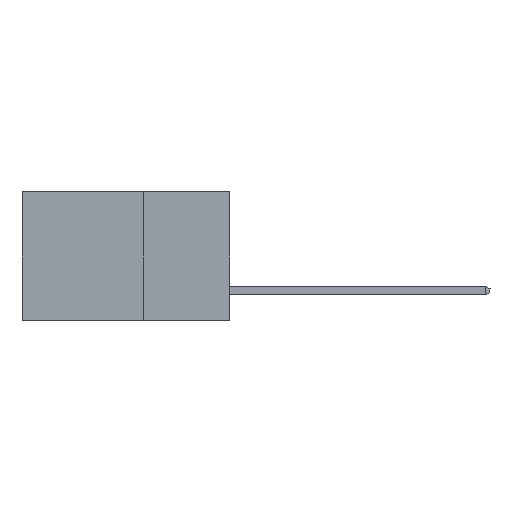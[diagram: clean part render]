
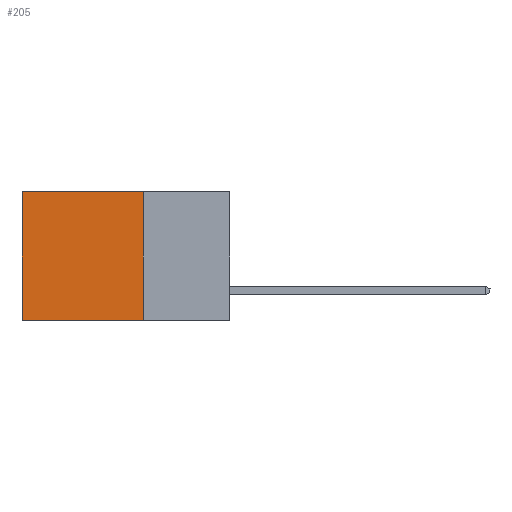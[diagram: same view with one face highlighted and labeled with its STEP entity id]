
A CAD part, left-side view. The second image highlights one B-rep face of the part: STEP entity #205.
In plain terms, the highlighted planar face has unit normal (-1, 0, 0).
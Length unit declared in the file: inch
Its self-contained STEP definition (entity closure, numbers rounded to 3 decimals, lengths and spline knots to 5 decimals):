
#205 = ADVANCED_FACE ( 'NONE', ( #17928 ), #16292, .F. ) ;
#658 = DIRECTION ( 'NONE',  ( 0., 0., -1. ) ) ;
#1501 = ORIENTED_EDGE ( 'NONE', *, *, #4145, .T. ) ;
#1997 = LINE ( 'NONE', #7866, #11590 ) ;
#3904 = LINE ( 'NONE', #15305, #12214 ) ;
#4145 = EDGE_CURVE ( 'NONE', #8951, #12545, #3904, .T. ) ;
#4415 = DIRECTION ( 'NONE',  ( 0., 1., 0. ) ) ;
#4969 = EDGE_CURVE ( 'NONE', #8951, #15960, #1997, .T. ) ;
#5435 = EDGE_CURVE ( 'NONE', #12545, #11303, #9252, .T. ) ;
#6039 = VECTOR ( 'NONE', #4415, 39.37008 ) ;
#6071 = CARTESIAN_POINT ( 'NONE',  ( 0.2615, 0.6, -0.37 ) ) ;
#6176 = CARTESIAN_POINT ( 'NONE',  ( 0.2615, 0.25, -0.37 ) ) ;
#6348 = DIRECTION ( 'NONE',  ( 0., 0., -1. ) ) ;
#7554 = CARTESIAN_POINT ( 'NONE',  ( 0.2615, 0.6, -0.37 ) ) ;
#7866 = CARTESIAN_POINT ( 'NONE',  ( 0.2615, 0.25, -0.37 ) ) ;
#8060 = VECTOR ( 'NONE', #15090, 39.37008 ) ;
#8951 = VERTEX_POINT ( 'NONE', #13808 ) ;
#9252 = LINE ( 'NONE', #7554, #8060 ) ;
#9755 = DIRECTION ( 'NONE',  ( 0., 1., 0. ) ) ;
#10037 = ORIENTED_EDGE ( 'NONE', *, *, #15325, .F. ) ;
#10166 = LINE ( 'NONE', #14853, #6039 ) ;
#11303 = VERTEX_POINT ( 'NONE', #6071 ) ;
#11590 = VECTOR ( 'NONE', #658, 39.37008 ) ;
#11899 = CARTESIAN_POINT ( 'NONE',  ( 0.2615, 0.6, 0. ) ) ;
#12176 = CARTESIAN_POINT ( 'NONE',  ( 0.2615, 0.25, -0.37 ) ) ;
#12214 = VECTOR ( 'NONE', #9755, 39.37008 ) ;
#12545 = VERTEX_POINT ( 'NONE', #11899 ) ;
#13386 = EDGE_LOOP ( 'NONE', ( #18352, #10037, #14983, #1501 ) ) ;
#13808 = CARTESIAN_POINT ( 'NONE',  ( 0.2615, 0.25, 0. ) ) ;
#14853 = CARTESIAN_POINT ( 'NONE',  ( 0.2615, 0.25, -0.37 ) ) ;
#14983 = ORIENTED_EDGE ( 'NONE', *, *, #4969, .F. ) ;
#15090 = DIRECTION ( 'NONE',  ( 0., 0., -1. ) ) ;
#15242 = DIRECTION ( 'NONE',  ( 1., 0., 0. ) ) ;
#15305 = CARTESIAN_POINT ( 'NONE',  ( 0.2615, 0.25, 0. ) ) ;
#15325 = EDGE_CURVE ( 'NONE', #15960, #11303, #10166, .T. ) ;
#15767 = AXIS2_PLACEMENT_3D ( 'NONE', #12176, #15242, #6348 ) ;
#15960 = VERTEX_POINT ( 'NONE', #6176 ) ;
#16292 = PLANE ( 'NONE',  #15767 ) ;
#17928 = FACE_OUTER_BOUND ( 'NONE', #13386, .T. ) ;
#18352 = ORIENTED_EDGE ( 'NONE', *, *, #5435, .T. ) ;
